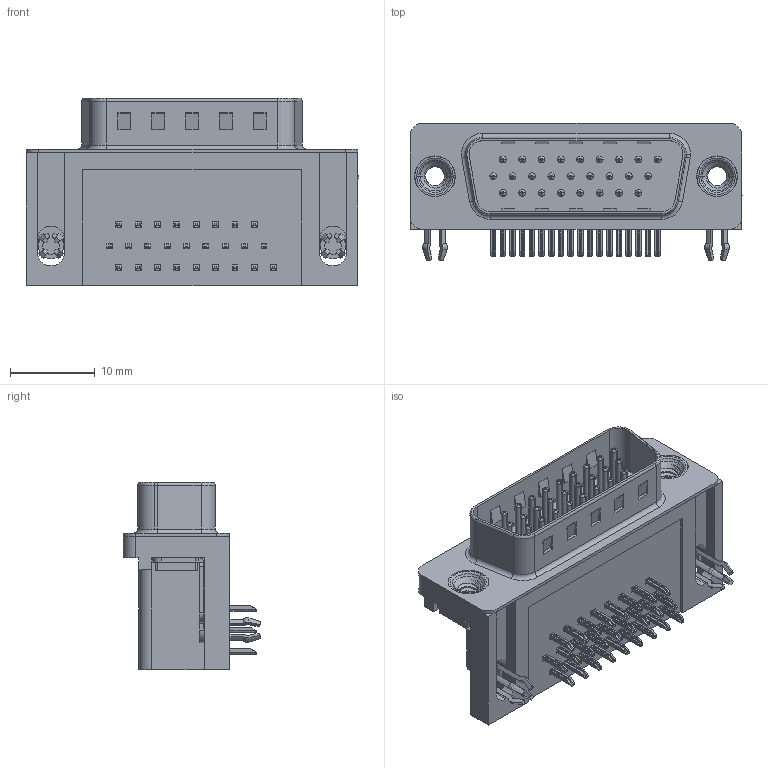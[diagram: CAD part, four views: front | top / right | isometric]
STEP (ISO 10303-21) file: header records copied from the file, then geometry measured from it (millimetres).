
FILE_DESCRIPTION (( 'STEP AP203' ), '1' );
FILE_NAME ('633-026-363-552.STEP', '2018-09-06T11:24:14', ( '' ), ( '' ), 'SwSTEP 2.0', 'SolidWorks 2016', '' );
FILE_SCHEMA (( 'CONFIG_CONTROL_DESIGN' ));
Length unit declared in the file: millimetre
Products named in the file (8): 633 Contact Middle; 633 Contact Top; 633 4 Prong Board Lock; 633 4-40 Threaded Rivet; 633-026-363-552; 633 Housing_26 Contact; 633 Shell_26 Contact; 633 Contact Bottom
Assembly tree (32 placements, depth 2):
  633-026-363-552
    633 Housing_26 Contact
    633 Shell_26 Contact
    633 Contact Bottom  x8
    633 Contact Middle  x9
    633 Contact Top  x9
    633 4 Prong Board Lock  x2
    633 4-40 Threaded Rivet  x2
Bounding box: 39.22 x 16.25 x 22.1 mm (x, y, z)
Volume: 5608.7 mm3; surface area: 7324.4 mm2
Topology: 32 solids, 32 shells, 2424 faces, 6054 edges, 3753 vertices
Faces by surface type: plane 1463, cylinder 684, torus 219, cone 52, bspline 6
Entity records: 25890 total; most frequent: CARTESIAN_POINT 5720, DIRECTION 4003, ORIENTED_EDGE 3798, EDGE_CURVE 1899, AXIS2_PLACEMENT_3D 1366, VECTOR 1271, LINE 1271, VERTEX_POINT 1217
